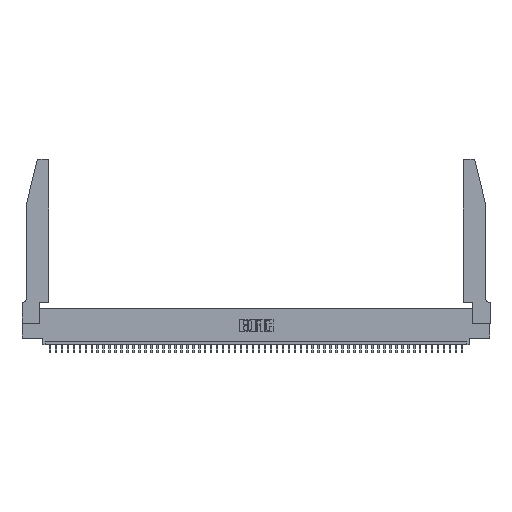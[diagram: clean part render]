
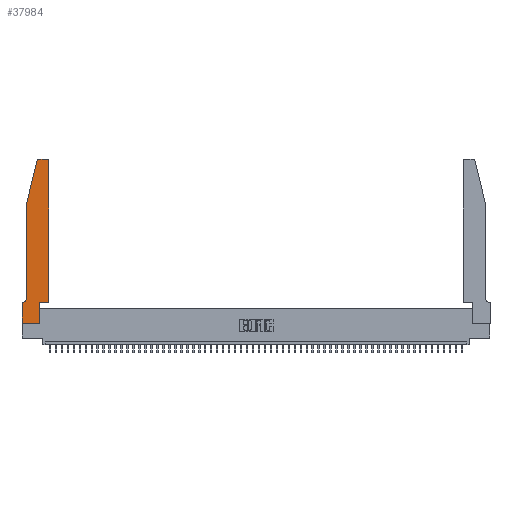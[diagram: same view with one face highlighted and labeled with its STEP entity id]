
A CAD part, top view. The second image highlights one B-rep face of the part: STEP entity #37984.
In plain terms, the highlighted planar face has unit normal (0, 0, 1).
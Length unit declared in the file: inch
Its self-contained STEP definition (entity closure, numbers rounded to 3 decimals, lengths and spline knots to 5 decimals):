
#99 = LINE ( 'NONE', #11969, #14354 ) ;
#923 = DIRECTION ( 'NONE',  ( 1., 0., 0. ) ) ;
#1076 = CARTESIAN_POINT ( 'NONE',  ( 0., 0.35, 0.37 ) ) ;
#2179 = DIRECTION ( 'NONE',  ( 0., 1., 0. ) ) ;
#3209 = CIRCLE ( 'NONE', #43817, 0.03 ) ;
#3218 = CARTESIAN_POINT ( 'NONE',  ( 0., 0., 0.37 ) ) ;
#3316 = VERTEX_POINT ( 'NONE', #18048 ) ;
#3409 = DIRECTION ( 'NONE',  ( -1., 0., 0. ) ) ;
#4101 = VERTEX_POINT ( 'NONE', #44052 ) ;
#5780 = DIRECTION ( 'NONE',  ( -1., 0., 0. ) ) ;
#6381 = CARTESIAN_POINT ( 'NONE',  ( 0.4505, 0.35, 0.37 ) ) ;
#6389 = DIRECTION ( 'NONE',  ( 1., 0., 0. ) ) ;
#6704 = CARTESIAN_POINT ( 'NONE',  ( 0., 0., 0.37 ) ) ;
#6954 = CIRCLE ( 'NONE', #53666, 0.03 ) ;
#7303 = LINE ( 'NONE', #12579, #46214 ) ;
#7483 = LINE ( 'NONE', #22856, #33462 ) ;
#9815 = LINE ( 'NONE', #19909, #14420 ) ;
#11647 = VERTEX_POINT ( 'NONE', #15764 ) ;
#11969 = CARTESIAN_POINT ( 'NONE',  ( 0.4505, 0.35, 0.37 ) ) ;
#12579 = CARTESIAN_POINT ( 'NONE',  ( 0., 0., 0.37 ) ) ;
#13362 = VERTEX_POINT ( 'NONE', #44381 ) ;
#14354 = VECTOR ( 'NONE', #15755, 39.37008 ) ;
#14420 = VECTOR ( 'NONE', #15705, 39.37008 ) ;
#15034 = EDGE_CURVE ( 'NONE', #3316, #13362, #35490, .T. ) ;
#15334 = VERTEX_POINT ( 'NONE', #21863 ) ;
#15705 = DIRECTION ( 'NONE',  ( -1., 0., 0. ) ) ;
#15755 = DIRECTION ( 'NONE',  ( 1., 0., 0. ) ) ;
#15764 = CARTESIAN_POINT ( 'NONE',  ( 0.25487, 2.72718, 0.37 ) ) ;
#15807 = DIRECTION ( 'NONE',  ( 0., -1., 0. ) ) ;
#17212 = VECTOR ( 'NONE', #38237, 39.37008 ) ;
#17859 = ORIENTED_EDGE ( 'NONE', *, *, #29421, .T. ) ;
#18035 = CARTESIAN_POINT ( 'NONE',  ( 0.284, 2.75, 0.37 ) ) ;
#18048 = CARTESIAN_POINT ( 'NONE',  ( 0.4505, 0.35, 0.37 ) ) ;
#18476 = EDGE_CURVE ( 'NONE', #20837, #32797, #9815, .T. ) ;
#18918 = DIRECTION ( 'NONE',  ( 0., 1., 0. ) ) ;
#18943 = ORIENTED_EDGE ( 'NONE', *, *, #44034, .T. ) ;
#19375 = EDGE_LOOP ( 'NONE', ( #29960, #50704, #17859, #18943, #22821, #41199, #26731, #37270, #25190, #19907, #35026, #39427 ) ) ;
#19907 = ORIENTED_EDGE ( 'NONE', *, *, #26597, .T. ) ;
#19909 = CARTESIAN_POINT ( 'NONE',  ( 0.2605, 2.75, 0.37 ) ) ;
#20056 = EDGE_CURVE ( 'NONE', #4101, #51827, #32509, .T. ) ;
#20837 = VERTEX_POINT ( 'NONE', #48703 ) ;
#21331 = EDGE_CURVE ( 'NONE', #45217, #27084, #36449, .T. ) ;
#21729 = LINE ( 'NONE', #46612, #17212 ) ;
#21863 = CARTESIAN_POINT ( 'NONE',  ( 0.0055, 0.35, 0.37 ) ) ;
#22821 = ORIENTED_EDGE ( 'NONE', *, *, #28015, .T. ) ;
#22856 = CARTESIAN_POINT ( 'NONE',  ( 0.0755, 2., 0.37 ) ) ;
#24728 = VECTOR ( 'NONE', #5780, 39.37008 ) ;
#24792 = AXIS2_PLACEMENT_3D ( 'NONE', #53018, #45249, #3409 ) ;
#25190 = ORIENTED_EDGE ( 'NONE', *, *, #21331, .T. ) ;
#26597 = EDGE_CURVE ( 'NONE', #27084, #3316, #99, .T. ) ;
#26613 = VECTOR ( 'NONE', #18918, 39.37008 ) ;
#26731 = ORIENTED_EDGE ( 'NONE', *, *, #20056, .T. ) ;
#27084 = VERTEX_POINT ( 'NONE', #49529 ) ;
#27818 = EDGE_CURVE ( 'NONE', #32797, #11647, #6954, .T. ) ;
#28015 = EDGE_CURVE ( 'NONE', #36707, #15334, #43973, .T. ) ;
#28818 = CARTESIAN_POINT ( 'NONE',  ( 0.0755, 2., 0.37 ) ) ;
#29421 = EDGE_CURVE ( 'NONE', #11647, #46004, #7483, .T. ) ;
#29960 = ORIENTED_EDGE ( 'NONE', *, *, #18476, .T. ) ;
#30545 = EDGE_CURVE ( 'NONE', #51827, #45217, #7303, .T. ) ;
#32269 = DIRECTION ( 'NONE',  ( 0., 0., 1. ) ) ;
#32368 = DIRECTION ( 'NONE',  ( 1., 0., 0. ) ) ;
#32509 = LINE ( 'NONE', #3218, #41557 ) ;
#32797 = VERTEX_POINT ( 'NONE', #18035 ) ;
#32992 = VECTOR ( 'NONE', #2179, 39.37008 ) ;
#33451 = DIRECTION ( 'NONE',  ( 1., 0., 0. ) ) ;
#33462 = VECTOR ( 'NONE', #52226, 39.37008 ) ;
#33737 = LINE ( 'NONE', #43065, #24728 ) ;
#34185 = EDGE_CURVE ( 'NONE', #13362, #20837, #3209, .T. ) ;
#34248 = PLANE ( 'NONE',  #48826 ) ;
#34303 = EDGE_CURVE ( 'NONE', #15334, #4101, #33737, .T. ) ;
#34677 = CARTESIAN_POINT ( 'NONE',  ( 0.2865, 0.35, 0.37 ) ) ;
#35026 = ORIENTED_EDGE ( 'NONE', *, *, #15034, .T. ) ;
#35490 = LINE ( 'NONE', #6381, #32992 ) ;
#36449 = LINE ( 'NONE', #34677, #26613 ) ;
#36707 = VERTEX_POINT ( 'NONE', #51414 ) ;
#37270 = ORIENTED_EDGE ( 'NONE', *, *, #30545, .T. ) ;
#37984 = ADVANCED_FACE ( 'NONE', ( #44515 ), #34248, .T. ) ;
#38237 = DIRECTION ( 'NONE',  ( 0., -1., 0. ) ) ;
#39427 = ORIENTED_EDGE ( 'NONE', *, *, #34185, .T. ) ;
#41199 = ORIENTED_EDGE ( 'NONE', *, *, #34303, .T. ) ;
#41557 = VECTOR ( 'NONE', #15807, 39.37008 ) ;
#43065 = CARTESIAN_POINT ( 'NONE',  ( 0.0755, 0.35, 0.37 ) ) ;
#43817 = AXIS2_PLACEMENT_3D ( 'NONE', #45276, #32269, #923 ) ;
#43973 = CIRCLE ( 'NONE', #24792, 0.07 ) ;
#44034 = EDGE_CURVE ( 'NONE', #46004, #36707, #21729, .T. ) ;
#44052 = CARTESIAN_POINT ( 'NONE',  ( 0., 0.35, 0.37 ) ) ;
#44381 = CARTESIAN_POINT ( 'NONE',  ( 0.4505, 2.72, 0.37 ) ) ;
#44515 = FACE_OUTER_BOUND ( 'NONE', #19375, .T. ) ;
#45217 = VERTEX_POINT ( 'NONE', #50334 ) ;
#45249 = DIRECTION ( 'NONE',  ( 0., 0., -1. ) ) ;
#45276 = CARTESIAN_POINT ( 'NONE',  ( 0.4205, 2.72, 0.37 ) ) ;
#46004 = VERTEX_POINT ( 'NONE', #28818 ) ;
#46214 = VECTOR ( 'NONE', #33451, 39.37008 ) ;
#46612 = CARTESIAN_POINT ( 'NONE',  ( 0.0755, 2., 0.37 ) ) ;
#48703 = CARTESIAN_POINT ( 'NONE',  ( 0.4205, 2.75, 0.37 ) ) ;
#48826 = AXIS2_PLACEMENT_3D ( 'NONE', #1076, #50555, #32368 ) ;
#49529 = CARTESIAN_POINT ( 'NONE',  ( 0.2865, 0.35, 0.37 ) ) ;
#50334 = CARTESIAN_POINT ( 'NONE',  ( 0.2865, 0., 0.37 ) ) ;
#50555 = DIRECTION ( 'NONE',  ( 0., 0., 1. ) ) ;
#50704 = ORIENTED_EDGE ( 'NONE', *, *, #27818, .T. ) ;
#51414 = CARTESIAN_POINT ( 'NONE',  ( 0.0755, 0.42, 0.37 ) ) ;
#51827 = VERTEX_POINT ( 'NONE', #6704 ) ;
#51959 = DIRECTION ( 'NONE',  ( 0., 0., 1. ) ) ;
#52226 = DIRECTION ( 'NONE',  ( -0.239, -0.971, 0. ) ) ;
#52542 = CARTESIAN_POINT ( 'NONE',  ( 0.284, 2.72, 0.37 ) ) ;
#53018 = CARTESIAN_POINT ( 'NONE',  ( 0.0055, 0.42, 0.37 ) ) ;
#53666 = AXIS2_PLACEMENT_3D ( 'NONE', #52542, #51959, #6389 ) ;
